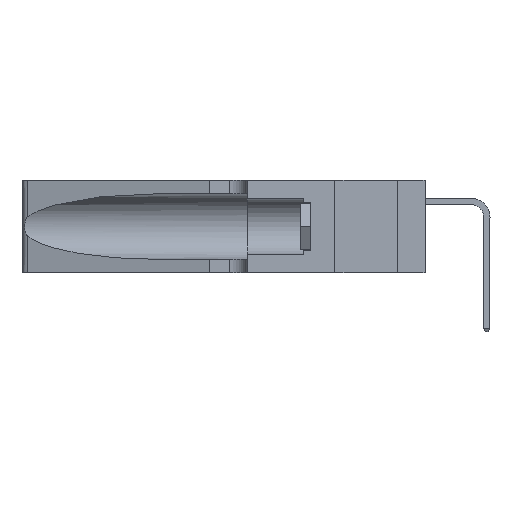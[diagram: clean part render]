
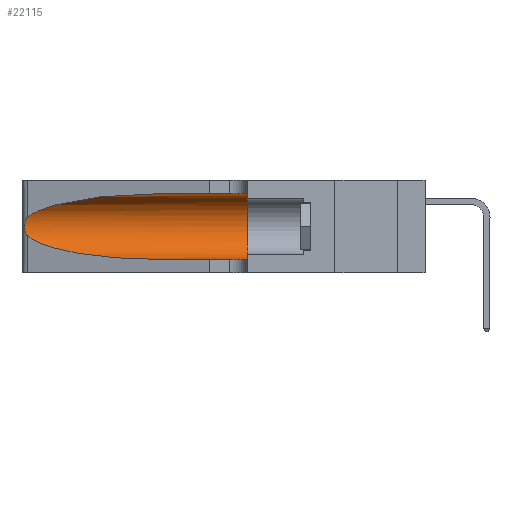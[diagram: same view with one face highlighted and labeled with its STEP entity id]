
A CAD part, left-side view. The second image highlights one B-rep face of the part: STEP entity #22115.
In plain terms, the highlighted cylindrical face has radius 3.308 mm (diameter 6.617 mm), a partial arc.
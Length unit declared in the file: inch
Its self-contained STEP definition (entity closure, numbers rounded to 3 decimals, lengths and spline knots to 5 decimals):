
#218 =( BOUNDED_CURVE ( )  B_SPLINE_CURVE ( 3, ( #4087, #22451, #6763, #25090 ),
 .UNSPECIFIED., .F., .T. ) 
 B_SPLINE_CURVE_WITH_KNOTS ( ( 4, 4 ),
 ( 3.44316, 4.71239 ),
 .UNSPECIFIED. ) 
 CURVE ( )  GEOMETRIC_REPRESENTATION_ITEM ( )  RATIONAL_B_SPLINE_CURVE ( ( 1., 0.87, 0.87, 1. ) ) 
 REPRESENTATION_ITEM ( '' )  );
#606 = CARTESIAN_POINT ( 'NONE',  ( 0.25555, 1.22993, 0.14849 ) ) ;
#826 = LINE ( 'NONE', #24109, #20943 ) ;
#842 = CARTESIAN_POINT ( 'NONE',  ( 0.1305, 0.35, 0.05475 ) ) ;
#1046 = DIRECTION ( 'NONE',  ( 0., -1., 0. ) ) ;
#1060 = CARTESIAN_POINT ( 'NONE',  ( 0.2373, 1.15595, 0.28018 ) ) ;
#1269 = DIRECTION ( 'NONE',  ( 0., -1., 0. ) ) ;
#2428 = B_SPLINE_CURVE_WITH_KNOTS ( 'NONE', 3,
 ( #31925, #24017, #21477, #5780, #24134, #8432, #26760, #11109, #29377, #13777, #32037, #16339, #606, #18954 ),
 .UNSPECIFIED., .F., .F.,
 ( 4, 2, 2, 2, 2, 2, 4 ),
 ( 0., 0.00027, 0.00053, 0.00107, 0.0016, 0.00187, 0.00214 ),
 .UNSPECIFIED. ) ;
#2489 = VERTEX_POINT ( 'NONE', #30105 ) ;
#2515 = EDGE_CURVE ( 'NONE', #2489, #31891, #218, .T. ) ;
#2736 = VERTEX_POINT ( 'NONE', #28612 ) ;
#4087 = CARTESIAN_POINT ( 'NONE',  ( 0.25487, 1.22718, 0.14631 ) ) ;
#5106 = ORIENTED_EDGE ( 'NONE', *, *, #31164, .F. ) ;
#5780 = CARTESIAN_POINT ( 'NONE',  ( 0.25787, 1.23484, 0.2124 ) ) ;
#6278 = DIRECTION ( 'NONE',  ( 0., 0., -1. ) ) ;
#6327 = CYLINDRICAL_SURFACE ( 'NONE', #15556, 0.13025 ) ;
#6763 = CARTESIAN_POINT ( 'NONE',  ( 0.18966, 0.96281, 0.05475 ) ) ;
#7159 = FACE_OUTER_BOUND ( 'NONE', #28943, .T. ) ;
#7404 = CIRCLE ( 'NONE', #29942, 0.13025 ) ;
#7617 = EDGE_CURVE ( 'NONE', #31891, #22634, #23962, .T. ) ;
#8432 = CARTESIAN_POINT ( 'NONE',  ( 0.26018, 1.23835, 0.19895 ) ) ;
#9918 = DIRECTION ( 'NONE',  ( 0., 1., 0. ) ) ;
#11109 = CARTESIAN_POINT ( 'NONE',  ( 0.26075, 1.23896, 0.178 ) ) ;
#12461 = VERTEX_POINT ( 'NONE', #32887 ) ;
#13777 = CARTESIAN_POINT ( 'NONE',  ( 0.25856, 1.23593, 0.16098 ) ) ;
#15556 = AXIS2_PLACEMENT_3D ( 'NONE', #16592, #21958, #6278 ) ;
#16339 = CARTESIAN_POINT ( 'NONE',  ( 0.25639, 1.23186, 0.15144 ) ) ;
#16592 = CARTESIAN_POINT ( 'NONE',  ( 0.1305, 1.61858, 0.185 ) ) ;
#17863 = ORIENTED_EDGE ( 'NONE', *, *, #26825, .T. ) ;
#18096 = EDGE_CURVE ( 'NONE', #12461, #2489, #2428, .T. ) ;
#18954 = CARTESIAN_POINT ( 'NONE',  ( 0.25487, 1.22718, 0.14631 ) ) ;
#19400 = CARTESIAN_POINT ( 'NONE',  ( 0.25487, 1.22718, 0.22369 ) ) ;
#19951 = VERTEX_POINT ( 'NONE', #22489 ) ;
#20943 = VECTOR ( 'NONE', #1046, 39.37008 ) ;
#21477 = CARTESIAN_POINT ( 'NONE',  ( 0.25639, 1.23184, 0.21858 ) ) ;
#21958 = DIRECTION ( 'NONE',  ( 0., -1., 0. ) ) ;
#22115 = ADVANCED_FACE ( 'NONE', ( #7159 ), #6327, .F. ) ;
#22451 = CARTESIAN_POINT ( 'NONE',  ( 0.2373, 1.15595, 0.08982 ) ) ;
#22489 = CARTESIAN_POINT ( 'NONE',  ( 0.1305, 0.35, 0.31525 ) ) ;
#22552 =( BOUNDED_CURVE ( )  B_SPLINE_CURVE ( 3, ( #24585, #27186, #1060, #19400 ),
 .UNSPECIFIED., .F., .T. ) 
 B_SPLINE_CURVE_WITH_KNOTS ( ( 4, 4 ),
 ( 1.5708, 2.84003 ),
 .UNSPECIFIED. ) 
 CURVE ( )  GEOMETRIC_REPRESENTATION_ITEM ( )  RATIONAL_B_SPLINE_CURVE ( ( 1., 0.87, 0.87, 1. ) ) 
 REPRESENTATION_ITEM ( '' )  );
#22634 = VERTEX_POINT ( 'NONE', #842 ) ;
#23962 = LINE ( 'NONE', #30024, #29262 ) ;
#24017 = CARTESIAN_POINT ( 'NONE',  ( 0.25555, 1.22994, 0.2215 ) ) ;
#24109 = CARTESIAN_POINT ( 'NONE',  ( 0.1305, 1.61858, 0.31525 ) ) ;
#24134 = CARTESIAN_POINT ( 'NONE',  ( 0.25854, 1.2359, 0.20912 ) ) ;
#24585 = CARTESIAN_POINT ( 'NONE',  ( 0.1305, 0.72297, 0.31525 ) ) ;
#25090 = CARTESIAN_POINT ( 'NONE',  ( 0.1305, 0.72297, 0.05475 ) ) ;
#25382 = ORIENTED_EDGE ( 'NONE', *, *, #18096, .T. ) ;
#25583 = CARTESIAN_POINT ( 'NONE',  ( 0.1305, 0.35, 0.185 ) ) ;
#25917 = ORIENTED_EDGE ( 'NONE', *, *, #7617, .T. ) ;
#26760 = CARTESIAN_POINT ( 'NONE',  ( 0.26075, 1.23896, 0.19203 ) ) ;
#26795 = ORIENTED_EDGE ( 'NONE', *, *, #31411, .F. ) ;
#26825 = EDGE_CURVE ( 'NONE', #2736, #12461, #22552, .T. ) ;
#27186 = CARTESIAN_POINT ( 'NONE',  ( 0.18966, 0.96281, 0.31525 ) ) ;
#28199 = DIRECTION ( 'NONE',  ( 0., 0., 1. ) ) ;
#28612 = CARTESIAN_POINT ( 'NONE',  ( 0.1305, 0.72297, 0.31525 ) ) ;
#28943 = EDGE_LOOP ( 'NONE', ( #17863, #25382, #29673, #25917, #26795, #5106 ) ) ;
#29262 = VECTOR ( 'NONE', #1269, 39.37008 ) ;
#29377 = CARTESIAN_POINT ( 'NONE',  ( 0.26017, 1.23833, 0.17102 ) ) ;
#29661 = CARTESIAN_POINT ( 'NONE',  ( 0.1305, 0.72297, 0.05475 ) ) ;
#29673 = ORIENTED_EDGE ( 'NONE', *, *, #2515, .T. ) ;
#29942 = AXIS2_PLACEMENT_3D ( 'NONE', #25583, #9918, #28199 ) ;
#30024 = CARTESIAN_POINT ( 'NONE',  ( 0.1305, 1.61858, 0.05475 ) ) ;
#30105 = CARTESIAN_POINT ( 'NONE',  ( 0.25487, 1.22718, 0.14631 ) ) ;
#31164 = EDGE_CURVE ( 'NONE', #2736, #19951, #826, .T. ) ;
#31411 = EDGE_CURVE ( 'NONE', #19951, #22634, #7404, .T. ) ;
#31891 = VERTEX_POINT ( 'NONE', #29661 ) ;
#31925 = CARTESIAN_POINT ( 'NONE',  ( 0.25487, 1.22718, 0.22369 ) ) ;
#32037 = CARTESIAN_POINT ( 'NONE',  ( 0.25789, 1.23486, 0.15765 ) ) ;
#32887 = CARTESIAN_POINT ( 'NONE',  ( 0.25487, 1.22718, 0.22369 ) ) ;
